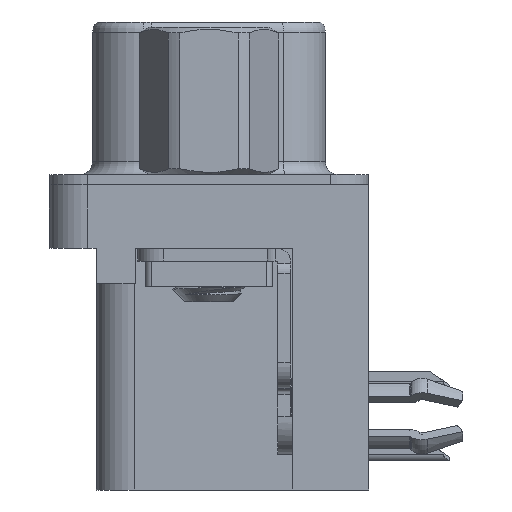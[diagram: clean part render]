
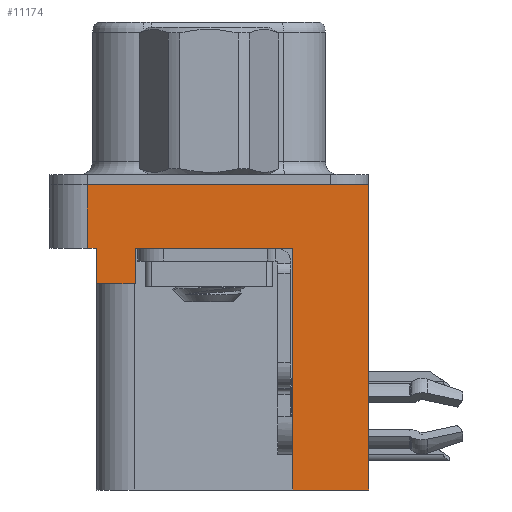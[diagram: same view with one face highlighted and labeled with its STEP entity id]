
A CAD part, left-side view. The second image highlights one B-rep face of the part: STEP entity #11174.
In plain terms, the highlighted planar face has unit normal (-1, 0, 0).
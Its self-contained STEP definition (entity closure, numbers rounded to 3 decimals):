
#42 = VECTOR ( 'NONE', #25898, 1000. ) ;
#322 = DIRECTION ( 'NONE',  ( 0., 0., 1. ) ) ;
#444 = LINE ( 'NONE', #23064, #21284 ) ;
#567 = EDGE_CURVE ( 'NONE', #7320, #8612, #2782, .T. ) ;
#984 = VERTEX_POINT ( 'NONE', #20073 ) ;
#992 = CARTESIAN_POINT ( 'NONE',  ( -2.935, 2.895, -3.9 ) ) ;
#1319 = ORIENTED_EDGE ( 'NONE', *, *, #13435, .F. ) ;
#1987 = EDGE_LOOP ( 'NONE', ( #2946, #7451, #9804, #18132, #19088, #11252, #12556, #3483, #1319, #15384 ) ) ;
#2163 = CARTESIAN_POINT ( 'NONE',  ( -2.935, -3.295, -2.5 ) ) ;
#2624 = FACE_OUTER_BOUND ( 'NONE', #1987, .T. ) ;
#2782 = LINE ( 'NONE', #18709, #11314 ) ;
#2946 = ORIENTED_EDGE ( 'NONE', *, *, #13773, .F. ) ;
#3154 = CARTESIAN_POINT ( 'NONE',  ( -2.935, -6.275, 0. ) ) ;
#3287 = EDGE_CURVE ( 'NONE', #5649, #7092, #8227, .T. ) ;
#3480 = VERTEX_POINT ( 'NONE', #18332 ) ;
#3483 = ORIENTED_EDGE ( 'NONE', *, *, #16108, .F. ) ;
#3571 = CARTESIAN_POINT ( 'NONE',  ( -2.935, -6.275, -2.5 ) ) ;
#3655 = DIRECTION ( 'NONE',  ( 0., 0., 1. ) ) ;
#3658 = LINE ( 'NONE', #14315, #9662 ) ;
#5304 = VERTEX_POINT ( 'NONE', #24401 ) ;
#5398 = VECTOR ( 'NONE', #12729, 1000. ) ;
#5649 = VERTEX_POINT ( 'NONE', #992 ) ;
#6109 = LINE ( 'NONE', #18489, #12137 ) ;
#7028 = CARTESIAN_POINT ( 'NONE',  ( -2.935, -6.275, -2.5 ) ) ;
#7092 = VERTEX_POINT ( 'NONE', #14172 ) ;
#7185 = DIRECTION ( 'NONE',  ( 0., -1., 0. ) ) ;
#7320 = VERTEX_POINT ( 'NONE', #25981 ) ;
#7437 = EDGE_CURVE ( 'NONE', #7092, #8612, #18683, .T. ) ;
#7451 = ORIENTED_EDGE ( 'NONE', *, *, #19863, .F. ) ;
#7807 = AXIS2_PLACEMENT_3D ( 'NONE', #7028, #19310, #10951 ) ;
#8213 = DIRECTION ( 'NONE',  ( 0., -1., 0. ) ) ;
#8227 = LINE ( 'NONE', #25168, #5398 ) ;
#8612 = VERTEX_POINT ( 'NONE', #11732 ) ;
#9106 = LINE ( 'NONE', #3154, #16361 ) ;
#9524 = VERTEX_POINT ( 'NONE', #13349 ) ;
#9662 = VECTOR ( 'NONE', #8213, 1000. ) ;
#9804 = ORIENTED_EDGE ( 'NONE', *, *, #567, .T. ) ;
#9927 = DIRECTION ( 'NONE',  ( 0., 1., 0. ) ) ;
#10951 = DIRECTION ( 'NONE',  ( 0., 0., 1. ) ) ;
#11025 = DIRECTION ( 'NONE',  ( 0., 0., 1. ) ) ;
#11035 = DIRECTION ( 'NONE',  ( 0., 0., 1. ) ) ;
#11174 = ADVANCED_FACE ( 'NONE', ( #2624 ), #17091, .T. ) ;
#11252 = ORIENTED_EDGE ( 'NONE', *, *, #18261, .T. ) ;
#11314 = VECTOR ( 'NONE', #22679, 1000. ) ;
#11732 = CARTESIAN_POINT ( 'NONE',  ( -2.935, 4.425, -2.5 ) ) ;
#12137 = VECTOR ( 'NONE', #322, 1000. ) ;
#12556 = ORIENTED_EDGE ( 'NONE', *, *, #19507, .T. ) ;
#12729 = DIRECTION ( 'NONE',  ( 0., 1., 0. ) ) ;
#13226 = VECTOR ( 'NONE', #11025, 1000. ) ;
#13349 = CARTESIAN_POINT ( 'NONE',  ( -2.935, 2.895, -2.5 ) ) ;
#13435 = EDGE_CURVE ( 'NONE', #984, #14899, #17727, .T. ) ;
#13773 = EDGE_CURVE ( 'NONE', #3480, #5304, #9106, .T. ) ;
#13968 = CARTESIAN_POINT ( 'NONE',  ( -2.935, -3.295, -12. ) ) ;
#14172 = CARTESIAN_POINT ( 'NONE',  ( -2.935, 4.425, -3.9 ) ) ;
#14315 = CARTESIAN_POINT ( 'NONE',  ( -2.935, -6.275, -2.5 ) ) ;
#14818 = LINE ( 'NONE', #23051, #13226 ) ;
#14899 = VERTEX_POINT ( 'NONE', #18454 ) ;
#15384 = ORIENTED_EDGE ( 'NONE', *, *, #22492, .T. ) ;
#15465 = VERTEX_POINT ( 'NONE', #2163 ) ;
#16108 = EDGE_CURVE ( 'NONE', #14899, #15465, #444, .T. ) ;
#16223 = VECTOR ( 'NONE', #3655, 1000. ) ;
#16361 = VECTOR ( 'NONE', #7185, 1000. ) ;
#17091 = PLANE ( 'NONE',  #7807 ) ;
#17727 = LINE ( 'NONE', #13968, #19325 ) ;
#18132 = ORIENTED_EDGE ( 'NONE', *, *, #7437, .F. ) ;
#18261 = EDGE_CURVE ( 'NONE', #5649, #9524, #14818, .T. ) ;
#18332 = CARTESIAN_POINT ( 'NONE',  ( -2.935, 4.775, 0. ) ) ;
#18454 = CARTESIAN_POINT ( 'NONE',  ( -2.935, -3.295, -12. ) ) ;
#18489 = CARTESIAN_POINT ( 'NONE',  ( -2.935, 4.775, -2.5 ) ) ;
#18683 = LINE ( 'NONE', #23860, #42 ) ;
#18709 = CARTESIAN_POINT ( 'NONE',  ( -2.935, -6.275, -2.5 ) ) ;
#19088 = ORIENTED_EDGE ( 'NONE', *, *, #3287, .F. ) ;
#19310 = DIRECTION ( 'NONE',  ( -1., 0., 0. ) ) ;
#19325 = VECTOR ( 'NONE', #9927, 1000. ) ;
#19507 = EDGE_CURVE ( 'NONE', #9524, #15465, #3658, .T. ) ;
#19863 = EDGE_CURVE ( 'NONE', #7320, #3480, #6109, .T. ) ;
#20073 = CARTESIAN_POINT ( 'NONE',  ( -2.935, -6.275, -12. ) ) ;
#21284 = VECTOR ( 'NONE', #11035, 1000. ) ;
#22492 = EDGE_CURVE ( 'NONE', #984, #5304, #24741, .T. ) ;
#22679 = DIRECTION ( 'NONE',  ( 0., -1., 0. ) ) ;
#23051 = CARTESIAN_POINT ( 'NONE',  ( -2.935, 2.895, -3.9 ) ) ;
#23064 = CARTESIAN_POINT ( 'NONE',  ( -2.935, -3.295, -12. ) ) ;
#23860 = CARTESIAN_POINT ( 'NONE',  ( -2.935, 4.425, -3.9 ) ) ;
#24401 = CARTESIAN_POINT ( 'NONE',  ( -2.935, -6.275, 0. ) ) ;
#24741 = LINE ( 'NONE', #3571, #16223 ) ;
#25168 = CARTESIAN_POINT ( 'NONE',  ( -2.935, 4.425, -3.9 ) ) ;
#25898 = DIRECTION ( 'NONE',  ( 0., 0., 1. ) ) ;
#25981 = CARTESIAN_POINT ( 'NONE',  ( -2.935, 4.775, -2.5 ) ) ;
